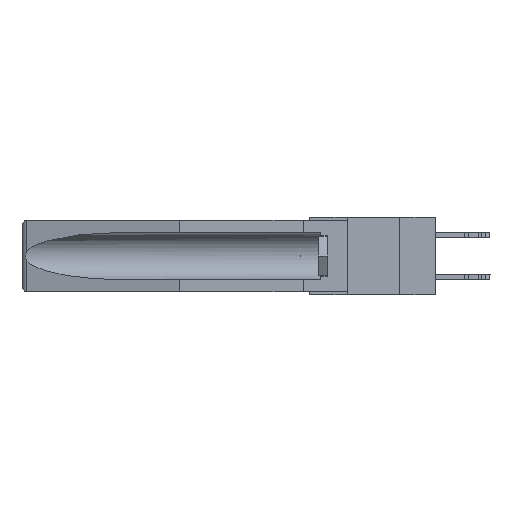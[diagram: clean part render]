
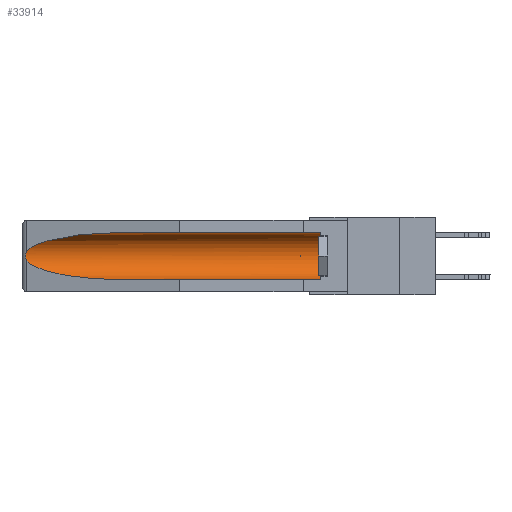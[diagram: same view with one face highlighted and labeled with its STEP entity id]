
A CAD part, left-side view. The second image highlights one B-rep face of the part: STEP entity #33914.
In plain terms, the highlighted cylindrical face has radius 2.857 mm (diameter 5.715 mm), a partial arc.
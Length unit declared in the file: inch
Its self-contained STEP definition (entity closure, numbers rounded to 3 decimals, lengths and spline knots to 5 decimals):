
#1395 = VERTEX_POINT ( 'NONE', #12580 ) ;
#2586 = CIRCLE ( 'NONE', #21518, 0.1125 ) ;
#3988 = CARTESIAN_POINT ( 'NONE',  ( 0.26537, 1.52718, -0.14972 ) ) ;
#4204 = VERTEX_POINT ( 'NONE', #19716 ) ;
#4214 = CARTESIAN_POINT ( 'NONE',  ( 0.26654, 1.53092, -0.15636 ) ) ;
#5338 = ORIENTED_EDGE ( 'NONE', *, *, #33956, .T. ) ;
#6130 = EDGE_CURVE ( 'NONE', #15310, #1395, #25388, .T. ) ;
#7490 = DIRECTION ( 'NONE',  ( 0., 1., 0. ) ) ;
#8684 = DIRECTION ( 'NONE',  ( 0., 1., 0. ) ) ;
#8868 = CARTESIAN_POINT ( 'NONE',  ( 0.25451, 1.48313, -0.24835 ) ) ;
#8939 = EDGE_CURVE ( 'NONE', #33112, #9840, #15812, .T. ) ;
#9840 = VERTEX_POINT ( 'NONE', #24681 ) ;
#9878 = EDGE_CURVE ( 'NONE', #21703, #4204, #29520, .T. ) ;
#11119 = EDGE_CURVE ( 'NONE', #9840, #4204, #13194, .T. ) ;
#12580 = CARTESIAN_POINT ( 'NONE',  ( 0.155, 1.07973, -0.059 ) ) ;
#12986 = CARTESIAN_POINT ( 'NONE',  ( 0.155, 0.126, -0.284 ) ) ;
#13007 = VECTOR ( 'NONE', #8684, 39.37008 ) ;
#13194 =( BOUNDED_CURVE ( )  B_SPLINE_CURVE ( 3, ( #14093, #8868, #22397, #33154 ),
 .UNSPECIFIED., .F., .F. ) 
 B_SPLINE_CURVE_WITH_KNOTS ( ( 4, 4 ),
 ( 0.1948, 1.5708 ),
 .UNSPECIFIED. ) 
 CURVE ( )  GEOMETRIC_REPRESENTATION_ITEM ( )  RATIONAL_B_SPLINE_CURVE ( ( 1., 0.848, 0.848, 1. ) ) 
 REPRESENTATION_ITEM ( '' )  );
#13298 = DIRECTION ( 'NONE',  ( 0., -1., 0. ) ) ;
#14093 = CARTESIAN_POINT ( 'NONE',  ( 0.26537, 1.52718, -0.19328 ) ) ;
#14683 = CARTESIAN_POINT ( 'NONE',  ( 0.26537, 1.52718, -0.19328 ) ) ;
#15073 = CARTESIAN_POINT ( 'NONE',  ( 0.25451, 1.48313, -0.09465 ) ) ;
#15200 = EDGE_LOOP ( 'NONE', ( #18786, #31021, #21037, #30301, #5338, #17700 ) ) ;
#15310 = VERTEX_POINT ( 'NONE', #17716 ) ;
#15812 = B_SPLINE_CURVE_WITH_KNOTS ( 'NONE', 3,
 ( #17796, #33846, #4214, #30762, #20145, #22732, #28169, #30877, #25561, #14683 ),
 .UNSPECIFIED., .F., .F.,
 ( 4, 2, 2, 2, 4 ),
 ( 0., 0.00029, 0.00058, 0.00087, 0.00117 ),
 .UNSPECIFIED. ) ;
#16081 = AXIS2_PLACEMENT_3D ( 'NONE', #21123, #7490, #26416 ) ;
#17214 = DIRECTION ( 'NONE',  ( 0., 1., 0. ) ) ;
#17486 = EDGE_CURVE ( 'NONE', #1395, #33112, #24267, .T. ) ;
#17700 = ORIENTED_EDGE ( 'NONE', *, *, #6130, .T. ) ;
#17716 = CARTESIAN_POINT ( 'NONE',  ( 0.155, 0.126, -0.059 ) ) ;
#17796 = CARTESIAN_POINT ( 'NONE',  ( 0.26537, 1.52718, -0.14972 ) ) ;
#18786 = ORIENTED_EDGE ( 'NONE', *, *, #17486, .T. ) ;
#19716 = CARTESIAN_POINT ( 'NONE',  ( 0.155, 1.07973, -0.284 ) ) ;
#20145 = CARTESIAN_POINT ( 'NONE',  ( 0.2675, 1.53308, -0.16763 ) ) ;
#20885 = CARTESIAN_POINT ( 'NONE',  ( 0.26537, 1.52718, -0.14972 ) ) ;
#21037 = ORIENTED_EDGE ( 'NONE', *, *, #11119, .T. ) ;
#21123 = CARTESIAN_POINT ( 'NONE',  ( 0.155, -0.30754, -0.1715 ) ) ;
#21518 = AXIS2_PLACEMENT_3D ( 'NONE', #24065, #13298, #32234 ) ;
#21703 = VERTEX_POINT ( 'NONE', #12986 ) ;
#21748 = CARTESIAN_POINT ( 'NONE',  ( 0.155, -0.30754, -0.284 ) ) ;
#22397 = CARTESIAN_POINT ( 'NONE',  ( 0.21114, 1.30732, -0.284 ) ) ;
#22517 = CYLINDRICAL_SURFACE ( 'NONE', #16081, 0.1125 ) ;
#22732 = CARTESIAN_POINT ( 'NONE',  ( 0.2675, 1.53308, -0.17534 ) ) ;
#23588 = CARTESIAN_POINT ( 'NONE',  ( 0.155, 1.07973, -0.059 ) ) ;
#24065 = CARTESIAN_POINT ( 'NONE',  ( 0.155, 0.126, -0.1715 ) ) ;
#24267 =( BOUNDED_CURVE ( )  B_SPLINE_CURVE ( 3, ( #23588, #28791, #15073, #20885 ),
 .UNSPECIFIED., .F., .F. ) 
 B_SPLINE_CURVE_WITH_KNOTS ( ( 4, 4 ),
 ( 4.71239, 6.08839 ),
 .UNSPECIFIED. ) 
 CURVE ( )  GEOMETRIC_REPRESENTATION_ITEM ( )  RATIONAL_B_SPLINE_CURVE ( ( 1., 0.848, 0.848, 1. ) ) 
 REPRESENTATION_ITEM ( '' )  );
#24681 = CARTESIAN_POINT ( 'NONE',  ( 0.26537, 1.52718, -0.19328 ) ) ;
#25388 = LINE ( 'NONE', #27709, #32143 ) ;
#25561 = CARTESIAN_POINT ( 'NONE',  ( 0.26597, 1.5296, -0.19026 ) ) ;
#26416 = DIRECTION ( 'NONE',  ( 0., 0., 1. ) ) ;
#27709 = CARTESIAN_POINT ( 'NONE',  ( 0.155, -0.30754, -0.059 ) ) ;
#28169 = CARTESIAN_POINT ( 'NONE',  ( 0.2673, 1.53269, -0.17917 ) ) ;
#28791 = CARTESIAN_POINT ( 'NONE',  ( 0.21114, 1.30732, -0.059 ) ) ;
#29520 = LINE ( 'NONE', #21748, #13007 ) ;
#30301 = ORIENTED_EDGE ( 'NONE', *, *, #9878, .F. ) ;
#30762 = CARTESIAN_POINT ( 'NONE',  ( 0.2673, 1.5327, -0.16383 ) ) ;
#30877 = CARTESIAN_POINT ( 'NONE',  ( 0.26655, 1.53094, -0.18657 ) ) ;
#31021 = ORIENTED_EDGE ( 'NONE', *, *, #8939, .T. ) ;
#32143 = VECTOR ( 'NONE', #17214, 39.37008 ) ;
#32234 = DIRECTION ( 'NONE',  ( 0., 0., 1. ) ) ;
#32258 = FACE_OUTER_BOUND ( 'NONE', #15200, .T. ) ;
#33112 = VERTEX_POINT ( 'NONE', #3988 ) ;
#33154 = CARTESIAN_POINT ( 'NONE',  ( 0.155, 1.07973, -0.284 ) ) ;
#33846 = CARTESIAN_POINT ( 'NONE',  ( 0.26597, 1.52961, -0.15275 ) ) ;
#33914 = ADVANCED_FACE ( 'NONE', ( #32258 ), #22517, .F. ) ;
#33956 = EDGE_CURVE ( 'NONE', #21703, #15310, #2586, .T. ) ;
